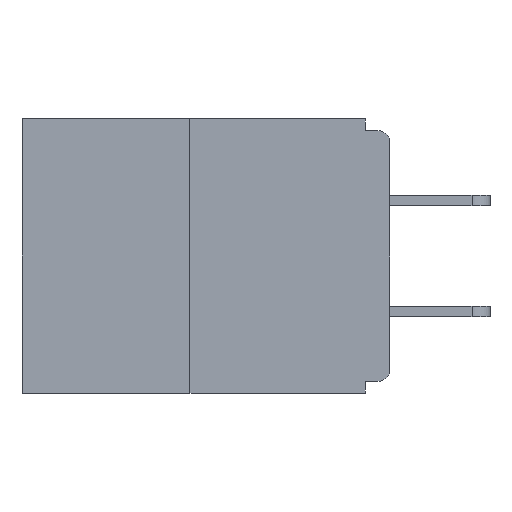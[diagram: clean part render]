
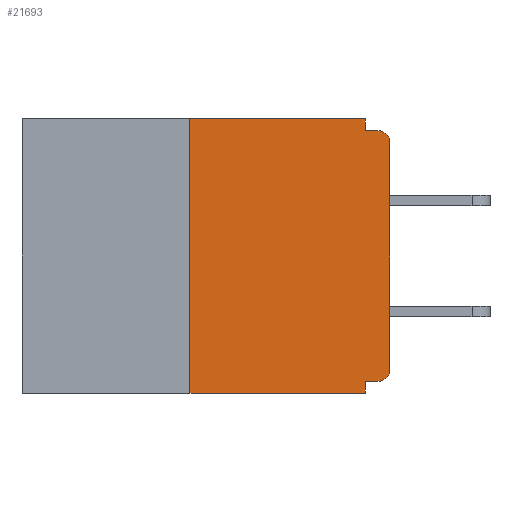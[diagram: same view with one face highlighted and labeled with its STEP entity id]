
A CAD part, left-side view. The second image highlights one B-rep face of the part: STEP entity #21693.
In plain terms, the highlighted planar face has unit normal (-1, 0, 0).
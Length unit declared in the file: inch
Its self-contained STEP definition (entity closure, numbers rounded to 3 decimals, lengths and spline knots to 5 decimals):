
#248 = LINE ( 'NONE', #1548, #18316 ) ;
#409 = CARTESIAN_POINT ( 'NONE',  ( 0., 0.25, -0.343 ) ) ;
#1101 = ORIENTED_EDGE ( 'NONE', *, *, #19618, .T. ) ;
#1181 = DIRECTION ( 'NONE',  ( 0., 0., -1. ) ) ;
#1548 = CARTESIAN_POINT ( 'NONE',  ( 0., 0.031, -0.343 ) ) ;
#1557 = CARTESIAN_POINT ( 'NONE',  ( 0., 0., -0.03 ) ) ;
#1709 = EDGE_CURVE ( 'NONE', #9615, #19071, #5737, .T. ) ;
#1881 = CARTESIAN_POINT ( 'NONE',  ( 0., 0., -0.015 ) ) ;
#1991 = ORIENTED_EDGE ( 'NONE', *, *, #3797, .F. ) ;
#2345 = FACE_OUTER_BOUND ( 'NONE', #15351, .T. ) ;
#2573 = CARTESIAN_POINT ( 'NONE',  ( 0., 0.25, 0. ) ) ;
#2950 = CIRCLE ( 'NONE', #16237, 0.015 ) ;
#3424 = EDGE_CURVE ( 'NONE', #10602, #8044, #6019, .T. ) ;
#3571 = CARTESIAN_POINT ( 'NONE',  ( 0., 0.031, -0.328 ) ) ;
#3797 = EDGE_CURVE ( 'NONE', #10016, #9805, #248, .T. ) ;
#3798 = ORIENTED_EDGE ( 'NONE', *, *, #1709, .T. ) ;
#3813 = VERTEX_POINT ( 'NONE', #4935 ) ;
#4935 = CARTESIAN_POINT ( 'NONE',  ( 0., 0.015, -0.015 ) ) ;
#5184 = EDGE_CURVE ( 'NONE', #13727, #3813, #18580, .T. ) ;
#5217 = ORIENTED_EDGE ( 'NONE', *, *, #5184, .F. ) ;
#5584 = VECTOR ( 'NONE', #23375, 39.37008 ) ;
#5634 = CARTESIAN_POINT ( 'NONE',  ( 0., 0.015, -0.328 ) ) ;
#5737 = LINE ( 'NONE', #26439, #7430 ) ;
#5853 = DIRECTION ( 'NONE',  ( -1., 0., 0. ) ) ;
#5885 = VERTEX_POINT ( 'NONE', #15566 ) ;
#5979 = CIRCLE ( 'NONE', #27480, 0.015 ) ;
#6019 = LINE ( 'NONE', #20075, #8367 ) ;
#6684 = LINE ( 'NONE', #17946, #19705 ) ;
#6787 = CARTESIAN_POINT ( 'NONE',  ( 0., 0.015, -0.03 ) ) ;
#7430 = VECTOR ( 'NONE', #24508, 39.37008 ) ;
#7828 = CARTESIAN_POINT ( 'NONE',  ( 0., 0.015, -0.313 ) ) ;
#8044 = VERTEX_POINT ( 'NONE', #2573 ) ;
#8367 = VECTOR ( 'NONE', #24338, 39.37008 ) ;
#8962 = DIRECTION ( 'NONE',  ( -1., 0., 0. ) ) ;
#9615 = VERTEX_POINT ( 'NONE', #12852 ) ;
#9667 = ORIENTED_EDGE ( 'NONE', *, *, #19276, .F. ) ;
#9805 = VERTEX_POINT ( 'NONE', #20068 ) ;
#10016 = VERTEX_POINT ( 'NONE', #3571 ) ;
#10602 = VERTEX_POINT ( 'NONE', #409 ) ;
#10634 = ORIENTED_EDGE ( 'NONE', *, *, #16220, .F. ) ;
#12524 = DIRECTION ( 'NONE',  ( 0., -1., 0. ) ) ;
#12559 = CARTESIAN_POINT ( 'NONE',  ( 0., 0.46, -0.343 ) ) ;
#12717 = CARTESIAN_POINT ( 'NONE',  ( 0., 0., -0.328 ) ) ;
#12852 = CARTESIAN_POINT ( 'NONE',  ( 0., 0., -0.313 ) ) ;
#13154 = DIRECTION ( 'NONE',  ( 0., 0., -1. ) ) ;
#13544 = VECTOR ( 'NONE', #12524, 39.37008 ) ;
#13727 = VERTEX_POINT ( 'NONE', #22329 ) ;
#14128 = DIRECTION ( 'NONE',  ( 1., 0., 0. ) ) ;
#14500 = DIRECTION ( 'NONE',  ( 0., 0., -1. ) ) ;
#14759 = DIRECTION ( 'NONE',  ( 0., -1., 0. ) ) ;
#14837 = ORIENTED_EDGE ( 'NONE', *, *, #19915, .T. ) ;
#15351 = EDGE_LOOP ( 'NONE', ( #23298, #21996, #18762, #1991, #10634, #1101, #3798, #14837, #5217, #9667 ) ) ;
#15566 = CARTESIAN_POINT ( 'NONE',  ( 0., 0.031, 0. ) ) ;
#16220 = EDGE_CURVE ( 'NONE', #18227, #10016, #16717, .T. ) ;
#16237 = AXIS2_PLACEMENT_3D ( 'NONE', #6787, #8962, #13154 ) ;
#16717 = LINE ( 'NONE', #12717, #17059 ) ;
#16805 = DIRECTION ( 'NONE',  ( 0., 0., -1. ) ) ;
#16839 = CARTESIAN_POINT ( 'NONE',  ( 0., 0.46, 0. ) ) ;
#17059 = VECTOR ( 'NONE', #26221, 39.37008 ) ;
#17262 = LINE ( 'NONE', #12559, #20376 ) ;
#17946 = CARTESIAN_POINT ( 'NONE',  ( 0., 0.031, 0. ) ) ;
#18021 = LINE ( 'NONE', #16839, #13544 ) ;
#18149 = DIRECTION ( 'NONE',  ( 0., 0., -1. ) ) ;
#18227 = VERTEX_POINT ( 'NONE', #5634 ) ;
#18316 = VECTOR ( 'NONE', #16805, 39.37008 ) ;
#18388 = PLANE ( 'NONE',  #20366 ) ;
#18580 = LINE ( 'NONE', #1881, #5584 ) ;
#18762 = ORIENTED_EDGE ( 'NONE', *, *, #22896, .T. ) ;
#19071 = VERTEX_POINT ( 'NONE', #1557 ) ;
#19276 = EDGE_CURVE ( 'NONE', #5885, #13727, #6684, .T. ) ;
#19618 = EDGE_CURVE ( 'NONE', #18227, #9615, #5979, .T. ) ;
#19705 = VECTOR ( 'NONE', #18149, 39.37008 ) ;
#19915 = EDGE_CURVE ( 'NONE', #19071, #3813, #2950, .T. ) ;
#20068 = CARTESIAN_POINT ( 'NONE',  ( 0., 0.031, -0.343 ) ) ;
#20075 = CARTESIAN_POINT ( 'NONE',  ( 0., 0.25, 0. ) ) ;
#20366 = AXIS2_PLACEMENT_3D ( 'NONE', #27014, #14128, #1181 ) ;
#20376 = VECTOR ( 'NONE', #14759, 39.37008 ) ;
#21385 = EDGE_CURVE ( 'NONE', #8044, #5885, #18021, .T. ) ;
#21693 = ADVANCED_FACE ( 'NONE', ( #2345 ), #18388, .F. ) ;
#21996 = ORIENTED_EDGE ( 'NONE', *, *, #3424, .F. ) ;
#22329 = CARTESIAN_POINT ( 'NONE',  ( 0., 0.031, -0.015 ) ) ;
#22896 = EDGE_CURVE ( 'NONE', #10602, #9805, #17262, .T. ) ;
#23298 = ORIENTED_EDGE ( 'NONE', *, *, #21385, .F. ) ;
#23375 = DIRECTION ( 'NONE',  ( 0., -1., 0. ) ) ;
#24338 = DIRECTION ( 'NONE',  ( 0., 0., 1. ) ) ;
#24508 = DIRECTION ( 'NONE',  ( 0., 0., 1. ) ) ;
#26221 = DIRECTION ( 'NONE',  ( 0., 1., 0. ) ) ;
#26439 = CARTESIAN_POINT ( 'NONE',  ( 0., 0., 0. ) ) ;
#27014 = CARTESIAN_POINT ( 'NONE',  ( 0., 0.46, 0. ) ) ;
#27480 = AXIS2_PLACEMENT_3D ( 'NONE', #7828, #5853, #14500 ) ;
